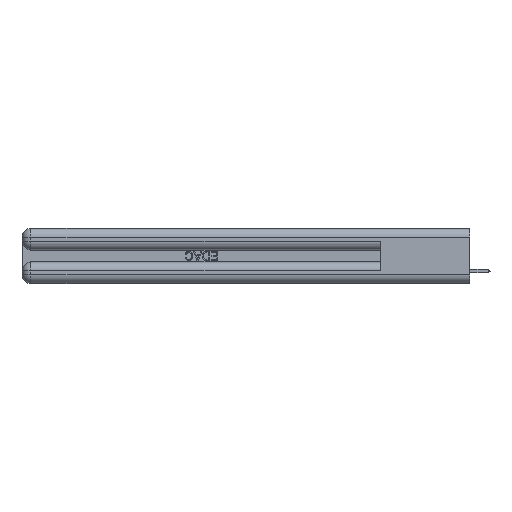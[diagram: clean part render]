
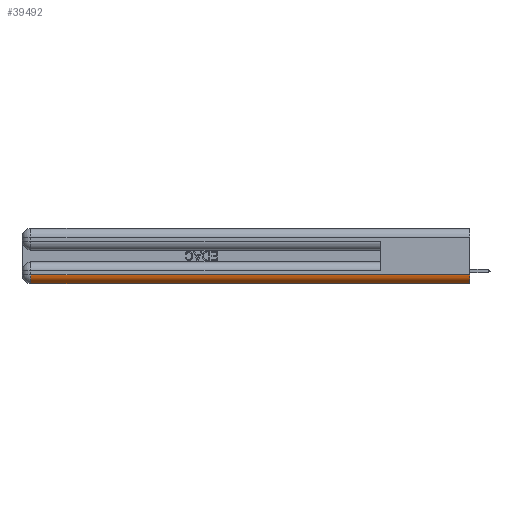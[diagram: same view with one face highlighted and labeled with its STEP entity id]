
A CAD part, left-side view. The second image highlights one B-rep face of the part: STEP entity #39492.
In plain terms, the highlighted cylindrical face has radius 1.524 mm (diameter 3.048 mm), a partial arc.
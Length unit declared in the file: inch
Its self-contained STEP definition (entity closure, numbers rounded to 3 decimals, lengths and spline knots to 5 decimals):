
#2810 = ORIENTED_EDGE ( 'NONE', *, *, #20327, .F. ) ;
#3573 = CYLINDRICAL_SURFACE ( 'NONE', #27577, 0.06 ) ;
#4009 = CARTESIAN_POINT ( 'NONE',  ( 0., 0., 0.06 ) ) ;
#4507 = ORIENTED_EDGE ( 'NONE', *, *, #11732, .F. ) ;
#5945 = DIRECTION ( 'NONE',  ( 0., -1., 0. ) ) ;
#6104 = DIRECTION ( 'NONE',  ( 0., 0., 1. ) ) ;
#6499 = DIRECTION ( 'NONE',  ( 0., 0., 1. ) ) ;
#7061 = EDGE_CURVE ( 'NONE', #13263, #22181, #53945, .T. ) ;
#9839 = CARTESIAN_POINT ( 'NONE',  ( 0.06, 0., 0.06 ) ) ;
#10090 = DIRECTION ( 'NONE',  ( 0., 1., 0. ) ) ;
#11732 = EDGE_CURVE ( 'NONE', #15119, #13263, #30703, .T. ) ;
#13263 = VERTEX_POINT ( 'NONE', #49691 ) ;
#14913 = CARTESIAN_POINT ( 'NONE',  ( 0.06, 2.94, 0.06 ) ) ;
#14996 = CARTESIAN_POINT ( 'NONE',  ( 0., 0., 0.06 ) ) ;
#15119 = VERTEX_POINT ( 'NONE', #48438 ) ;
#16567 = CARTESIAN_POINT ( 'NONE',  ( 0.06, 3., 0. ) ) ;
#20201 = VECTOR ( 'NONE', #50506, 39.37008 ) ;
#20327 = EDGE_CURVE ( 'NONE', #22181, #42302, #32230, .T. ) ;
#22106 = LINE ( 'NONE', #16567, #20201 ) ;
#22181 = VERTEX_POINT ( 'NONE', #4009 ) ;
#23660 = ORIENTED_EDGE ( 'NONE', *, *, #7061, .F. ) ;
#27577 = AXIS2_PLACEMENT_3D ( 'NONE', #9839, #52089, #32865 ) ;
#28115 = EDGE_LOOP ( 'NONE', ( #2810, #23660, #4507, #51983 ) ) ;
#28227 = EDGE_CURVE ( 'NONE', #42302, #15119, #22106, .T. ) ;
#28790 = AXIS2_PLACEMENT_3D ( 'NONE', #14913, #10090, #6104 ) ;
#30528 = AXIS2_PLACEMENT_3D ( 'NONE', #31741, #5945, #6499 ) ;
#30703 = CIRCLE ( 'NONE', #28790, 0.06 ) ;
#31741 = CARTESIAN_POINT ( 'NONE',  ( 0.06, 0., 0.06 ) ) ;
#32230 = CIRCLE ( 'NONE', #30528, 0.06 ) ;
#32865 = DIRECTION ( 'NONE',  ( 0., 0., 1. ) ) ;
#36234 = DIRECTION ( 'NONE',  ( 0., -1., 0. ) ) ;
#39492 = ADVANCED_FACE ( 'NONE', ( #43798 ), #3573, .T. ) ;
#42302 = VERTEX_POINT ( 'NONE', #54335 ) ;
#43798 = FACE_OUTER_BOUND ( 'NONE', #28115, .T. ) ;
#48000 = VECTOR ( 'NONE', #36234, 39.37008 ) ;
#48438 = CARTESIAN_POINT ( 'NONE',  ( 0.06, 2.94, 0. ) ) ;
#49691 = CARTESIAN_POINT ( 'NONE',  ( 0., 2.94, 0.06 ) ) ;
#50506 = DIRECTION ( 'NONE',  ( 0., 1., 0. ) ) ;
#51983 = ORIENTED_EDGE ( 'NONE', *, *, #28227, .F. ) ;
#52089 = DIRECTION ( 'NONE',  ( 0., 1., 0. ) ) ;
#53945 = LINE ( 'NONE', #14996, #48000 ) ;
#54335 = CARTESIAN_POINT ( 'NONE',  ( 0.06, 0., 0. ) ) ;
